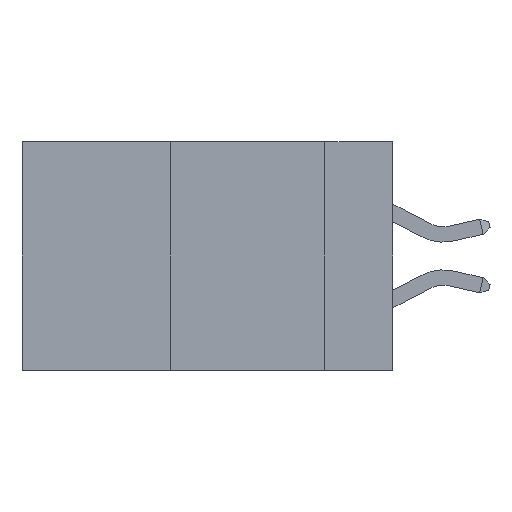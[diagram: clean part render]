
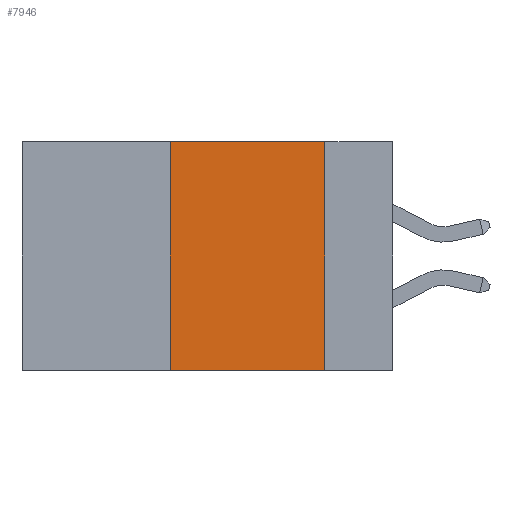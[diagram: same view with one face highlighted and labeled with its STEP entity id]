
A CAD part, left-side view. The second image highlights one B-rep face of the part: STEP entity #7946.
In plain terms, the highlighted planar face has unit normal (-1, 0, 0).
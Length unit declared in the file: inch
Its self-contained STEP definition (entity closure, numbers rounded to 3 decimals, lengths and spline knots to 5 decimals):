
#948 = EDGE_CURVE ( 'NONE', #31139, #31389, #31174, .T. ) ;
#1244 = LINE ( 'NONE', #29563, #21349 ) ;
#1739 = PLANE ( 'NONE',  #4800 ) ;
#3623 = DIRECTION ( 'NONE',  ( 0., 0., 1. ) ) ;
#4800 = AXIS2_PLACEMENT_3D ( 'NONE', #22831, #25795, #7136 ) ;
#5732 = LINE ( 'NONE', #19380, #33280 ) ;
#7136 = DIRECTION ( 'NONE',  ( 0., 0., -1. ) ) ;
#7340 = LINE ( 'NONE', #12568, #11007 ) ;
#7946 = ADVANCED_FACE ( 'NONE', ( #24621 ), #1739, .F. ) ;
#8290 = DIRECTION ( 'NONE',  ( 0., -1., 0. ) ) ;
#8598 = CARTESIAN_POINT ( 'NONE',  ( 0., 0.11, -0.37 ) ) ;
#10007 = CARTESIAN_POINT ( 'NONE',  ( 0., 0.36, -0.37 ) ) ;
#11007 = VECTOR ( 'NONE', #22656, 39.37008 ) ;
#12568 = CARTESIAN_POINT ( 'NONE',  ( 0., 0.11, 0. ) ) ;
#12589 = EDGE_LOOP ( 'NONE', ( #31699, #18218, #16581, #15507 ) ) ;
#13863 = DIRECTION ( 'NONE',  ( 0., -1., 0. ) ) ;
#15410 = EDGE_CURVE ( 'NONE', #31139, #22405, #5732, .T. ) ;
#15507 = ORIENTED_EDGE ( 'NONE', *, *, #948, .T. ) ;
#16581 = ORIENTED_EDGE ( 'NONE', *, *, #15410, .F. ) ;
#18218 = ORIENTED_EDGE ( 'NONE', *, *, #25904, .F. ) ;
#19380 = CARTESIAN_POINT ( 'NONE',  ( 0., 0.36, 0. ) ) ;
#20133 = VERTEX_POINT ( 'NONE', #25719 ) ;
#21349 = VECTOR ( 'NONE', #13863, 39.37008 ) ;
#22405 = VERTEX_POINT ( 'NONE', #30710 ) ;
#22656 = DIRECTION ( 'NONE',  ( 0., 0., -1. ) ) ;
#22831 = CARTESIAN_POINT ( 'NONE',  ( 0., 0.6, 0. ) ) ;
#24621 = FACE_OUTER_BOUND ( 'NONE', #12589, .T. ) ;
#25719 = CARTESIAN_POINT ( 'NONE',  ( 0., 0.11, 0. ) ) ;
#25795 = DIRECTION ( 'NONE',  ( 1., 0., 0. ) ) ;
#25840 = CARTESIAN_POINT ( 'NONE',  ( 0., 0.6, -0.37 ) ) ;
#25904 = EDGE_CURVE ( 'NONE', #22405, #20133, #1244, .T. ) ;
#26971 = EDGE_CURVE ( 'NONE', #20133, #31389, #7340, .T. ) ;
#29516 = VECTOR ( 'NONE', #8290, 39.37008 ) ;
#29563 = CARTESIAN_POINT ( 'NONE',  ( 0., 0.6, 0. ) ) ;
#30710 = CARTESIAN_POINT ( 'NONE',  ( 0., 0.36, 0. ) ) ;
#31139 = VERTEX_POINT ( 'NONE', #10007 ) ;
#31174 = LINE ( 'NONE', #25840, #29516 ) ;
#31389 = VERTEX_POINT ( 'NONE', #8598 ) ;
#31699 = ORIENTED_EDGE ( 'NONE', *, *, #26971, .F. ) ;
#33280 = VECTOR ( 'NONE', #3623, 39.37008 ) ;
